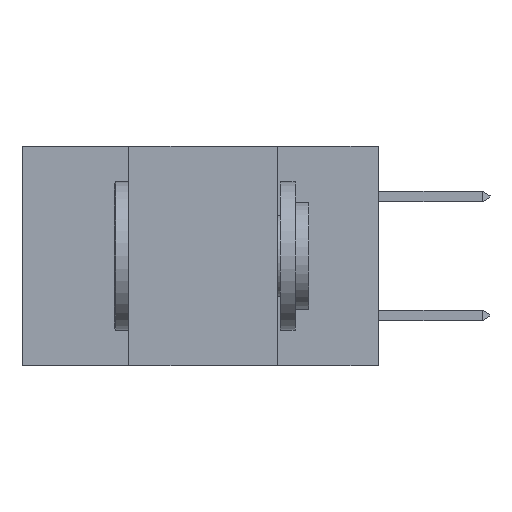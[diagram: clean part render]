
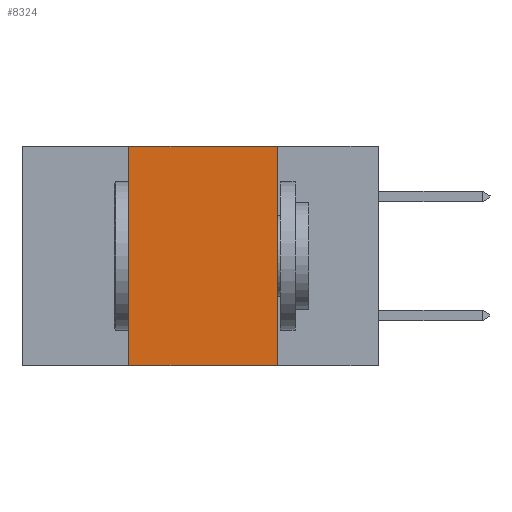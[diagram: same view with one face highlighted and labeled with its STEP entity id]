
A CAD part, left-side view. The second image highlights one B-rep face of the part: STEP entity #8324.
In plain terms, the highlighted planar face has unit normal (-1, 0, 0).
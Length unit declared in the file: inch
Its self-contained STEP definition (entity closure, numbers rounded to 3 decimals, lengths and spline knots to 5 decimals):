
#357 = ORIENTED_EDGE ( 'NONE', *, *, #2166, .F. ) ;
#891 = LINE ( 'NONE', #12781, #11662 ) ;
#1637 = CARTESIAN_POINT ( 'NONE',  ( 0., 0.6, 0. ) ) ;
#2098 = ORIENTED_EDGE ( 'NONE', *, *, #5998, .F. ) ;
#2166 = EDGE_CURVE ( 'NONE', #16001, #2591, #11635, .T. ) ;
#2307 = VECTOR ( 'NONE', #10253, 39.37008 ) ;
#2455 = LINE ( 'NONE', #11379, #2307 ) ;
#2591 = VERTEX_POINT ( 'NONE', #13118 ) ;
#2649 = VECTOR ( 'NONE', #15350, 39.37008 ) ;
#2824 = VERTEX_POINT ( 'NONE', #5857 ) ;
#2846 = CARTESIAN_POINT ( 'NONE',  ( 0., 0.42, -0.37 ) ) ;
#2876 = EDGE_CURVE ( 'NONE', #8579, #2591, #2455, .T. ) ;
#4238 = FACE_OUTER_BOUND ( 'NONE', #15184, .T. ) ;
#4850 = ORIENTED_EDGE ( 'NONE', *, *, #2876, .T. ) ;
#5645 = PLANE ( 'NONE',  #13477 ) ;
#5857 = CARTESIAN_POINT ( 'NONE',  ( 0., 0.42, 0. ) ) ;
#5998 = EDGE_CURVE ( 'NONE', #8579, #2824, #12568, .T. ) ;
#6124 = CARTESIAN_POINT ( 'NONE',  ( 0., 0.17, -0.37 ) ) ;
#8233 = DIRECTION ( 'NONE',  ( 1., 0., 0. ) ) ;
#8324 = ADVANCED_FACE ( 'NONE', ( #4238 ), #5645, .F. ) ;
#8579 = VERTEX_POINT ( 'NONE', #2846 ) ;
#10172 = DIRECTION ( 'NONE',  ( 0., 0., -1. ) ) ;
#10253 = DIRECTION ( 'NONE',  ( 0., -1., 0. ) ) ;
#11139 = DIRECTION ( 'NONE',  ( 0., -1., 0. ) ) ;
#11379 = CARTESIAN_POINT ( 'NONE',  ( 0., 0.6, -0.37 ) ) ;
#11625 = CARTESIAN_POINT ( 'NONE',  ( 0., 0.42, -0.37 ) ) ;
#11635 = LINE ( 'NONE', #6124, #12009 ) ;
#11662 = VECTOR ( 'NONE', #11139, 39.37008 ) ;
#12009 = VECTOR ( 'NONE', #10172, 39.37008 ) ;
#12568 = LINE ( 'NONE', #11625, #2649 ) ;
#12781 = CARTESIAN_POINT ( 'NONE',  ( 0., 0.6, 0. ) ) ;
#13118 = CARTESIAN_POINT ( 'NONE',  ( 0., 0.17, -0.37 ) ) ;
#13199 = ORIENTED_EDGE ( 'NONE', *, *, #14501, .F. ) ;
#13477 = AXIS2_PLACEMENT_3D ( 'NONE', #1637, #8233, #15958 ) ;
#14501 = EDGE_CURVE ( 'NONE', #2824, #16001, #891, .T. ) ;
#15184 = EDGE_LOOP ( 'NONE', ( #357, #13199, #2098, #4850 ) ) ;
#15350 = DIRECTION ( 'NONE',  ( 0., 0., 1. ) ) ;
#15958 = DIRECTION ( 'NONE',  ( 0., 0., -1. ) ) ;
#16001 = VERTEX_POINT ( 'NONE', #16311 ) ;
#16311 = CARTESIAN_POINT ( 'NONE',  ( 0., 0.17, 0. ) ) ;
